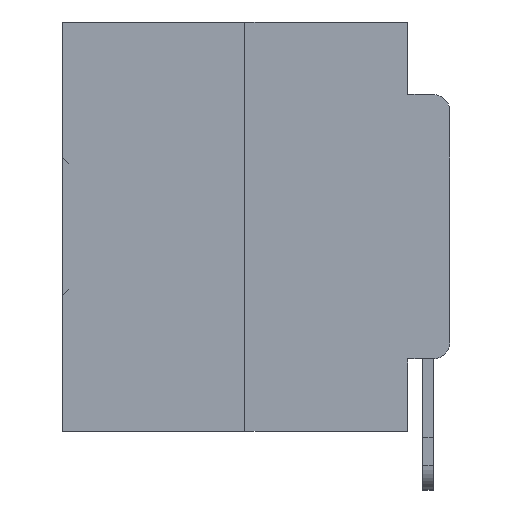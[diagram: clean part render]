
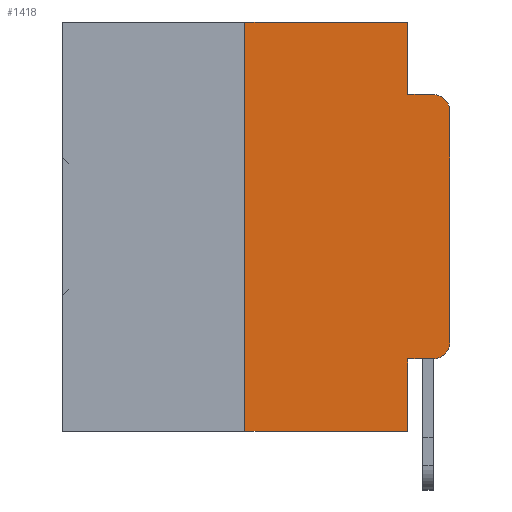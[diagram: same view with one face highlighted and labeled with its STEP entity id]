
A CAD part, left-side view. The second image highlights one B-rep face of the part: STEP entity #1418.
In plain terms, the highlighted planar face has unit normal (-1, 0, 0).
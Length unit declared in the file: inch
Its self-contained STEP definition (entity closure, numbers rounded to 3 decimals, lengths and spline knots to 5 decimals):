
#137 = VERTEX_POINT ( 'NONE', #4870 ) ;
#702 = ORIENTED_EDGE ( 'NONE', *, *, #8931, .T. ) ;
#1418 = ADVANCED_FACE ( 'NONE', ( #1473 ), #1644, .F. ) ;
#1473 = FACE_OUTER_BOUND ( 'NONE', #20647, .T. ) ;
#1644 = PLANE ( 'NONE',  #23842 ) ;
#2208 = DIRECTION ( 'NONE',  ( 0., 0., -1. ) ) ;
#2486 = VECTOR ( 'NONE', #9634, 39.37008 ) ;
#2837 = VERTEX_POINT ( 'NONE', #21928 ) ;
#3216 = VERTEX_POINT ( 'NONE', #26613 ) ;
#3550 = VERTEX_POINT ( 'NONE', #5711 ) ;
#3848 = CARTESIAN_POINT ( 'NONE',  ( 0., 0.25, 0. ) ) ;
#4492 = LINE ( 'NONE', #22755, #32972 ) ;
#4595 = CARTESIAN_POINT ( 'NONE',  ( 0., 0.02, -0.3915 ) ) ;
#4854 = LINE ( 'NONE', #8342, #30698 ) ;
#4870 = CARTESIAN_POINT ( 'NONE',  ( 0., 0., -0.3915 ) ) ;
#5227 = DIRECTION ( 'NONE',  ( 0., -1., 0. ) ) ;
#5348 = ORIENTED_EDGE ( 'NONE', *, *, #35456, .F. ) ;
#5711 = CARTESIAN_POINT ( 'NONE',  ( 0., 0.02, -0.0885 ) ) ;
#6253 = DIRECTION ( 'NONE',  ( 0., 0., 1. ) ) ;
#6627 = DIRECTION ( 'NONE',  ( 0., 0., 1. ) ) ;
#7220 = DIRECTION ( 'NONE',  ( 1., 0., 0. ) ) ;
#7396 = DIRECTION ( 'NONE',  ( 0., 0., -1. ) ) ;
#7767 = CARTESIAN_POINT ( 'NONE',  ( 0., 0.051, 0. ) ) ;
#8342 = CARTESIAN_POINT ( 'NONE',  ( 0., 0.473, 0. ) ) ;
#8931 = EDGE_CURVE ( 'NONE', #26758, #20430, #9209, .T. ) ;
#9201 = VERTEX_POINT ( 'NONE', #32611 ) ;
#9209 = LINE ( 'NONE', #32565, #15646 ) ;
#9524 = ORIENTED_EDGE ( 'NONE', *, *, #33638, .F. ) ;
#9634 = DIRECTION ( 'NONE',  ( 0., -1., 0. ) ) ;
#9654 = EDGE_CURVE ( 'NONE', #3216, #137, #17693, .T. ) ;
#9670 = VERTEX_POINT ( 'NONE', #12909 ) ;
#10907 = VERTEX_POINT ( 'NONE', #35295 ) ;
#12314 = EDGE_CURVE ( 'NONE', #9201, #20430, #29548, .T. ) ;
#12370 = EDGE_CURVE ( 'NONE', #9201, #3216, #33468, .T. ) ;
#12909 = CARTESIAN_POINT ( 'NONE',  ( 0., 0., -0.1085 ) ) ;
#13444 = ORIENTED_EDGE ( 'NONE', *, *, #29994, .T. ) ;
#14840 = AXIS2_PLACEMENT_3D ( 'NONE', #31813, #15289, #34604 ) ;
#14908 = VECTOR ( 'NONE', #2208, 39.37008 ) ;
#15289 = DIRECTION ( 'NONE',  ( -1., 0., 0. ) ) ;
#15646 = VECTOR ( 'NONE', #21567, 39.37008 ) ;
#15929 = CARTESIAN_POINT ( 'NONE',  ( 0., 0.051, 0. ) ) ;
#16818 = CARTESIAN_POINT ( 'NONE',  ( 0., 0.25, -0.5 ) ) ;
#16853 = VECTOR ( 'NONE', #6627, 39.37008 ) ;
#16860 = ORIENTED_EDGE ( 'NONE', *, *, #12314, .F. ) ;
#17693 = CIRCLE ( 'NONE', #21349, 0.02 ) ;
#18814 = DIRECTION ( 'NONE',  ( 0., 0., -1. ) ) ;
#19409 = DIRECTION ( 'NONE',  ( 0., -1., 0. ) ) ;
#19632 = VECTOR ( 'NONE', #5227, 39.37008 ) ;
#20430 = VERTEX_POINT ( 'NONE', #28858 ) ;
#20647 = EDGE_LOOP ( 'NONE', ( #35806, #13444, #5348, #9524, #33426, #24980, #702, #16860, #31626, #25749 ) ) ;
#21349 = AXIS2_PLACEMENT_3D ( 'NONE', #4595, #23881, #7396 ) ;
#21567 = DIRECTION ( 'NONE',  ( 0., -1., 0. ) ) ;
#21928 = CARTESIAN_POINT ( 'NONE',  ( 0., 0.25, 0. ) ) ;
#22755 = CARTESIAN_POINT ( 'NONE',  ( 0., 0., 0. ) ) ;
#23839 = VECTOR ( 'NONE', #18814, 39.37008 ) ;
#23842 = AXIS2_PLACEMENT_3D ( 'NONE', #26362, #7220, #26480 ) ;
#23881 = DIRECTION ( 'NONE',  ( -1., 0., 0. ) ) ;
#24202 = LINE ( 'NONE', #3848, #16853 ) ;
#24434 = EDGE_CURVE ( 'NONE', #137, #9670, #4492, .T. ) ;
#24980 = ORIENTED_EDGE ( 'NONE', *, *, #28120, .F. ) ;
#25593 = EDGE_CURVE ( 'NONE', #2837, #31761, #4854, .T. ) ;
#25749 = ORIENTED_EDGE ( 'NONE', *, *, #9654, .T. ) ;
#26129 = CARTESIAN_POINT ( 'NONE',  ( 0., 0.051, -0.0885 ) ) ;
#26362 = CARTESIAN_POINT ( 'NONE',  ( 0., 0.473, 0. ) ) ;
#26480 = DIRECTION ( 'NONE',  ( 0., 0., -1. ) ) ;
#26613 = CARTESIAN_POINT ( 'NONE',  ( 0., 0.02, -0.4115 ) ) ;
#26758 = VERTEX_POINT ( 'NONE', #16818 ) ;
#28120 = EDGE_CURVE ( 'NONE', #26758, #2837, #24202, .T. ) ;
#28858 = CARTESIAN_POINT ( 'NONE',  ( 0., 0.051, -0.5 ) ) ;
#29548 = LINE ( 'NONE', #15929, #14908 ) ;
#29994 = EDGE_CURVE ( 'NONE', #9670, #3550, #34063, .T. ) ;
#30013 = CARTESIAN_POINT ( 'NONE',  ( 0., 0.051, -0.4115 ) ) ;
#30057 = LINE ( 'NONE', #26129, #2486 ) ;
#30698 = VECTOR ( 'NONE', #19409, 39.37008 ) ;
#31082 = CARTESIAN_POINT ( 'NONE',  ( 0., 0.051, 0. ) ) ;
#31164 = LINE ( 'NONE', #7767, #23839 ) ;
#31626 = ORIENTED_EDGE ( 'NONE', *, *, #12370, .T. ) ;
#31761 = VERTEX_POINT ( 'NONE', #31082 ) ;
#31813 = CARTESIAN_POINT ( 'NONE',  ( 0., 0.02, -0.1085 ) ) ;
#32565 = CARTESIAN_POINT ( 'NONE',  ( 0., 0.473, -0.5 ) ) ;
#32611 = CARTESIAN_POINT ( 'NONE',  ( 0., 0.051, -0.4115 ) ) ;
#32972 = VECTOR ( 'NONE', #6253, 39.37008 ) ;
#33426 = ORIENTED_EDGE ( 'NONE', *, *, #25593, .F. ) ;
#33468 = LINE ( 'NONE', #30013, #19632 ) ;
#33638 = EDGE_CURVE ( 'NONE', #31761, #10907, #31164, .T. ) ;
#34063 = CIRCLE ( 'NONE', #14840, 0.02 ) ;
#34604 = DIRECTION ( 'NONE',  ( 0., 0., -1. ) ) ;
#35295 = CARTESIAN_POINT ( 'NONE',  ( 0., 0.051, -0.0885 ) ) ;
#35456 = EDGE_CURVE ( 'NONE', #10907, #3550, #30057, .T. ) ;
#35806 = ORIENTED_EDGE ( 'NONE', *, *, #24434, .T. ) ;
